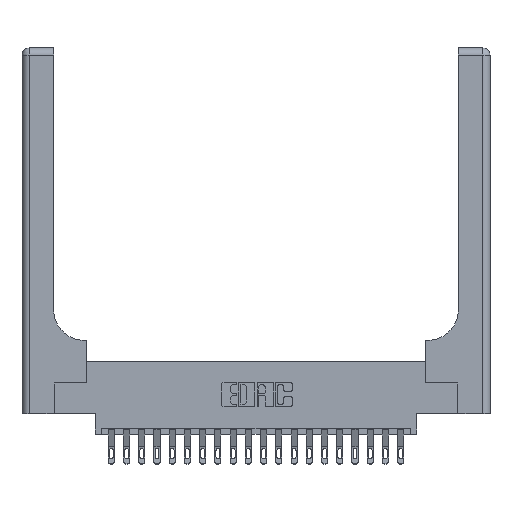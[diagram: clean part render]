
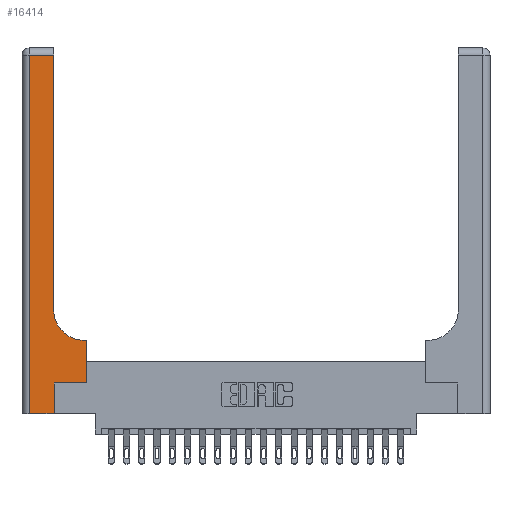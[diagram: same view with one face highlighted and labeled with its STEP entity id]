
A CAD part, top view. The second image highlights one B-rep face of the part: STEP entity #16414.
In plain terms, the highlighted planar face has unit normal (0, 0, 1).
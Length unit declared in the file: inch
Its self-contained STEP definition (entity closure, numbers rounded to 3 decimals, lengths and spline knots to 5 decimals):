
#37 = CARTESIAN_POINT ( 'NONE',  ( 0.26, 0.85, 0.37 ) ) ;
#419 = ORIENTED_EDGE ( 'NONE', *, *, #13299, .T. ) ;
#889 = CARTESIAN_POINT ( 'NONE',  ( 0.26, 2.94, 0.37 ) ) ;
#929 = EDGE_CURVE ( 'NONE', #5298, #6798, #7085, .T. ) ;
#1108 = EDGE_LOOP ( 'NONE', ( #419, #9348, #9890, #3047, #7493, #7730, #16606, #8276, #14263 ) ) ;
#1628 = VERTEX_POINT ( 'NONE', #18171 ) ;
#1722 = CARTESIAN_POINT ( 'NONE',  ( 0.528, 0.6, 0.37 ) ) ;
#1888 = CARTESIAN_POINT ( 'NONE',  ( 0.26, 3., 0.37 ) ) ;
#1982 = AXIS2_PLACEMENT_3D ( 'NONE', #13781, #3767, #15459 ) ;
#2295 = LINE ( 'NONE', #21473, #19566 ) ;
#2623 = VECTOR ( 'NONE', #4981, 39.37008 ) ;
#3032 = DIRECTION ( 'NONE',  ( 0., -1., 0. ) ) ;
#3047 = ORIENTED_EDGE ( 'NONE', *, *, #14802, .T. ) ;
#3353 = LINE ( 'NONE', #14264, #7274 ) ;
#3439 = EDGE_CURVE ( 'NONE', #10601, #1628, #3353, .T. ) ;
#3493 = CARTESIAN_POINT ( 'NONE',  ( 0.528, 0.25, 0.37 ) ) ;
#3767 = DIRECTION ( 'NONE',  ( 0., 0., -1. ) ) ;
#4301 = LINE ( 'NONE', #1888, #21036 ) ;
#4410 = VECTOR ( 'NONE', #14551, 39.37008 ) ;
#4590 = CARTESIAN_POINT ( 'NONE',  ( 0.26, 0.6, 0.37 ) ) ;
#4832 = DIRECTION ( 'NONE',  ( 1., 0., 0. ) ) ;
#4981 = DIRECTION ( 'NONE',  ( -1., 0., 0. ) ) ;
#5298 = VERTEX_POINT ( 'NONE', #889 ) ;
#6798 = VERTEX_POINT ( 'NONE', #16544 ) ;
#6894 = LINE ( 'NONE', #16501, #19175 ) ;
#7085 = LINE ( 'NONE', #11632, #2623 ) ;
#7274 = VECTOR ( 'NONE', #19235, 39.37008 ) ;
#7493 = ORIENTED_EDGE ( 'NONE', *, *, #3439, .T. ) ;
#7513 = VECTOR ( 'NONE', #3032, 39.37008 ) ;
#7544 = CARTESIAN_POINT ( 'NONE',  ( 0.51, 0.6, 0.37 ) ) ;
#7617 = PLANE ( 'NONE',  #16840 ) ;
#7730 = ORIENTED_EDGE ( 'NONE', *, *, #11088, .T. ) ;
#8276 = ORIENTED_EDGE ( 'NONE', *, *, #17295, .T. ) ;
#9348 = ORIENTED_EDGE ( 'NONE', *, *, #929, .T. ) ;
#9466 = VECTOR ( 'NONE', #11382, 39.37008 ) ;
#9890 = ORIENTED_EDGE ( 'NONE', *, *, #11868, .T. ) ;
#10030 = VERTEX_POINT ( 'NONE', #37 ) ;
#10261 = DIRECTION ( 'NONE',  ( 0., 1., 0. ) ) ;
#10601 = VERTEX_POINT ( 'NONE', #18287 ) ;
#10928 = VERTEX_POINT ( 'NONE', #7544 ) ;
#10980 = DIRECTION ( 'NONE',  ( -1., 0., 0. ) ) ;
#11037 = CARTESIAN_POINT ( 'NONE',  ( 0.06, 0., 0.37 ) ) ;
#11088 = EDGE_CURVE ( 'NONE', #1628, #20570, #17200, .T. ) ;
#11382 = DIRECTION ( 'NONE',  ( -1., 0., 0. ) ) ;
#11632 = CARTESIAN_POINT ( 'NONE',  ( 0., 2.94, 0.37 ) ) ;
#11868 = EDGE_CURVE ( 'NONE', #6798, #15222, #20316, .T. ) ;
#13299 = EDGE_CURVE ( 'NONE', #10030, #5298, #4301, .T. ) ;
#13781 = CARTESIAN_POINT ( 'NONE',  ( 0.51, 0.85, 0.37 ) ) ;
#13886 = LINE ( 'NONE', #4590, #9466 ) ;
#14217 = CIRCLE ( 'NONE', #1982, 0.25 ) ;
#14263 = ORIENTED_EDGE ( 'NONE', *, *, #15611, .T. ) ;
#14264 = CARTESIAN_POINT ( 'NONE',  ( 0.265, 0., 0.37 ) ) ;
#14551 = DIRECTION ( 'NONE',  ( 1., 0., 0. ) ) ;
#14802 = EDGE_CURVE ( 'NONE', #15222, #10601, #6894, .T. ) ;
#14816 = DIRECTION ( 'NONE',  ( 0., 1., 0. ) ) ;
#15222 = VERTEX_POINT ( 'NONE', #11037 ) ;
#15459 = DIRECTION ( 'NONE',  ( 1., 0., 0. ) ) ;
#15495 = VERTEX_POINT ( 'NONE', #1722 ) ;
#15611 = EDGE_CURVE ( 'NONE', #10928, #10030, #14217, .T. ) ;
#16414 = ADVANCED_FACE ( 'NONE', ( #20191 ), #7617, .F. ) ;
#16501 = CARTESIAN_POINT ( 'NONE',  ( 0., 0., 0.37 ) ) ;
#16544 = CARTESIAN_POINT ( 'NONE',  ( 0.06, 2.94, 0.37 ) ) ;
#16606 = ORIENTED_EDGE ( 'NONE', *, *, #18750, .T. ) ;
#16840 = AXIS2_PLACEMENT_3D ( 'NONE', #19294, #20976, #10980 ) ;
#17200 = LINE ( 'NONE', #17891, #4410 ) ;
#17295 = EDGE_CURVE ( 'NONE', #15495, #10928, #13886, .T. ) ;
#17891 = CARTESIAN_POINT ( 'NONE',  ( 0.265, 0.25, 0.37 ) ) ;
#18171 = CARTESIAN_POINT ( 'NONE',  ( 0.265, 0.25, 0.37 ) ) ;
#18287 = CARTESIAN_POINT ( 'NONE',  ( 0.265, 0., 0.37 ) ) ;
#18750 = EDGE_CURVE ( 'NONE', #20570, #15495, #2295, .T. ) ;
#19175 = VECTOR ( 'NONE', #4832, 39.37008 ) ;
#19235 = DIRECTION ( 'NONE',  ( 0., 1., 0. ) ) ;
#19294 = CARTESIAN_POINT ( 'NONE',  ( 0., 3., 0.37 ) ) ;
#19566 = VECTOR ( 'NONE', #14816, 39.37008 ) ;
#19708 = CARTESIAN_POINT ( 'NONE',  ( 0.06, 3., 0.37 ) ) ;
#20191 = FACE_OUTER_BOUND ( 'NONE', #1108, .T. ) ;
#20316 = LINE ( 'NONE', #19708, #7513 ) ;
#20570 = VERTEX_POINT ( 'NONE', #3493 ) ;
#20976 = DIRECTION ( 'NONE',  ( 0., 0., -1. ) ) ;
#21036 = VECTOR ( 'NONE', #10261, 39.37008 ) ;
#21473 = CARTESIAN_POINT ( 'NONE',  ( 0.528, 0.25, 0.37 ) ) ;
